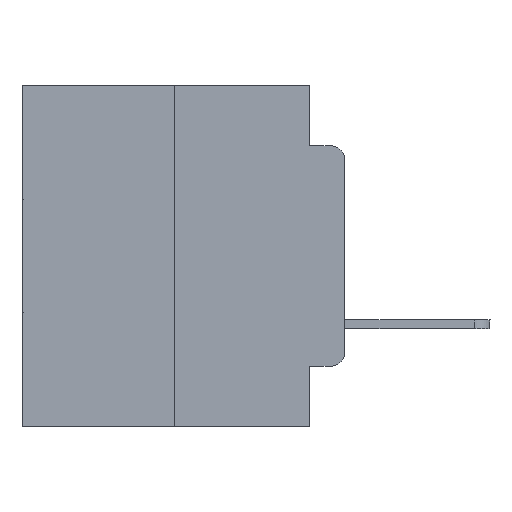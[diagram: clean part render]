
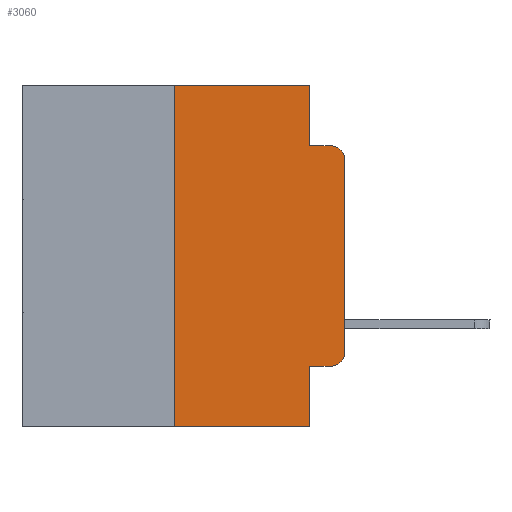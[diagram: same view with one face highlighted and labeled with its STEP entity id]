
A CAD part, left-side view. The second image highlights one B-rep face of the part: STEP entity #3060.
In plain terms, the highlighted planar face has unit normal (-1, 0, 0).
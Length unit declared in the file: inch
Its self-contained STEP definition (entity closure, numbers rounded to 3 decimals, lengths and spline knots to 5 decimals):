
#223 = DIRECTION ( 'NONE',  ( -1., 0., 0. ) ) ;
#539 = CARTESIAN_POINT ( 'NONE',  ( 0., 0.051, -0.0885 ) ) ;
#551 = VERTEX_POINT ( 'NONE', #13104 ) ;
#1118 = VERTEX_POINT ( 'NONE', #13674 ) ;
#1303 = DIRECTION ( 'NONE',  ( 0., -1., 0. ) ) ;
#1791 = CARTESIAN_POINT ( 'NONE',  ( 0., 0.25, 0. ) ) ;
#2303 = VERTEX_POINT ( 'NONE', #17810 ) ;
#2354 = VERTEX_POINT ( 'NONE', #6662 ) ;
#2661 = DIRECTION ( 'NONE',  ( 0., 0., -1. ) ) ;
#2842 = ORIENTED_EDGE ( 'NONE', *, *, #4212, .T. ) ;
#2928 = VECTOR ( 'NONE', #25773, 39.37008 ) ;
#2979 = EDGE_CURVE ( 'NONE', #2354, #1118, #25266, .T. ) ;
#3060 = ADVANCED_FACE ( 'NONE', ( #3319 ), #23708, .F. ) ;
#3319 = FACE_OUTER_BOUND ( 'NONE', #12115, .T. ) ;
#3343 = LINE ( 'NONE', #13105, #24347 ) ;
#3654 = VECTOR ( 'NONE', #1303, 39.37008 ) ;
#3935 = DIRECTION ( 'NONE',  ( 0., -1., 0. ) ) ;
#4157 = VECTOR ( 'NONE', #12078, 39.37008 ) ;
#4212 = EDGE_CURVE ( 'NONE', #8080, #551, #16313, .T. ) ;
#4447 = ORIENTED_EDGE ( 'NONE', *, *, #25679, .T. ) ;
#4883 = EDGE_CURVE ( 'NONE', #2303, #24372, #14687, .T. ) ;
#5353 = CARTESIAN_POINT ( 'NONE',  ( 0., 0.473, -0.5 ) ) ;
#5866 = CARTESIAN_POINT ( 'NONE',  ( 0., 0.051, -0.0885 ) ) ;
#6138 = ORIENTED_EDGE ( 'NONE', *, *, #2979, .F. ) ;
#6162 = DIRECTION ( 'NONE',  ( 0., 0., -1. ) ) ;
#6662 = CARTESIAN_POINT ( 'NONE',  ( 0., 0.051, -0.4115 ) ) ;
#6898 = DIRECTION ( 'NONE',  ( 0., 0., -1. ) ) ;
#8073 = CARTESIAN_POINT ( 'NONE',  ( 0., 0.473, 0. ) ) ;
#8080 = VERTEX_POINT ( 'NONE', #8433 ) ;
#8363 = AXIS2_PLACEMENT_3D ( 'NONE', #21636, #25627, #21457 ) ;
#8419 = CARTESIAN_POINT ( 'NONE',  ( 0., 0.02, -0.3915 ) ) ;
#8433 = CARTESIAN_POINT ( 'NONE',  ( 0., 0.02, -0.4115 ) ) ;
#8574 = CARTESIAN_POINT ( 'NONE',  ( 0., 0., -0.1085 ) ) ;
#8920 = ORIENTED_EDGE ( 'NONE', *, *, #13687, .T. ) ;
#9030 = ORIENTED_EDGE ( 'NONE', *, *, #18184, .F. ) ;
#9921 = VECTOR ( 'NONE', #12457, 39.37008 ) ;
#10866 = ORIENTED_EDGE ( 'NONE', *, *, #4883, .F. ) ;
#11330 = ORIENTED_EDGE ( 'NONE', *, *, #13579, .T. ) ;
#11761 = CARTESIAN_POINT ( 'NONE',  ( 0., 0.02, -0.0885 ) ) ;
#11883 = AXIS2_PLACEMENT_3D ( 'NONE', #8419, #223, #6162 ) ;
#11957 = LINE ( 'NONE', #17740, #3654 ) ;
#12078 = DIRECTION ( 'NONE',  ( 0., 0., 1. ) ) ;
#12115 = EDGE_LOOP ( 'NONE', ( #11330, #4447, #24808, #23043, #10866, #9030, #8920, #6138, #24757, #2842 ) ) ;
#12457 = DIRECTION ( 'NONE',  ( 0., -1., 0. ) ) ;
#12649 = EDGE_CURVE ( 'NONE', #24372, #23539, #3343, .T. ) ;
#13104 = CARTESIAN_POINT ( 'NONE',  ( 0., 0., -0.3915 ) ) ;
#13105 = CARTESIAN_POINT ( 'NONE',  ( 0., 0.051, 0. ) ) ;
#13303 = CIRCLE ( 'NONE', #8363, 0.02 ) ;
#13579 = EDGE_CURVE ( 'NONE', #551, #26294, #24578, .T. ) ;
#13674 = CARTESIAN_POINT ( 'NONE',  ( 0., 0.051, -0.5 ) ) ;
#13687 = EDGE_CURVE ( 'NONE', #20233, #1118, #21127, .T. ) ;
#14687 = LINE ( 'NONE', #8073, #9921 ) ;
#15639 = CARTESIAN_POINT ( 'NONE',  ( 0., 0.473, 0. ) ) ;
#15775 = CARTESIAN_POINT ( 'NONE',  ( 0., 0., 0. ) ) ;
#16161 = AXIS2_PLACEMENT_3D ( 'NONE', #15639, #25661, #19357 ) ;
#16313 = CIRCLE ( 'NONE', #11883, 0.02 ) ;
#16830 = LINE ( 'NONE', #5866, #21285 ) ;
#17740 = CARTESIAN_POINT ( 'NONE',  ( 0., 0.051, -0.4115 ) ) ;
#17810 = CARTESIAN_POINT ( 'NONE',  ( 0., 0.25, 0. ) ) ;
#18184 = EDGE_CURVE ( 'NONE', #20233, #2303, #22641, .T. ) ;
#18734 = VERTEX_POINT ( 'NONE', #11761 ) ;
#19357 = DIRECTION ( 'NONE',  ( 0., 0., -1. ) ) ;
#19499 = DIRECTION ( 'NONE',  ( 0., 0., 1. ) ) ;
#19988 = CARTESIAN_POINT ( 'NONE',  ( 0., 0.25, -0.5 ) ) ;
#20225 = VECTOR ( 'NONE', #2661, 39.37008 ) ;
#20233 = VERTEX_POINT ( 'NONE', #19988 ) ;
#21127 = LINE ( 'NONE', #5353, #2928 ) ;
#21285 = VECTOR ( 'NONE', #3935, 39.37008 ) ;
#21297 = EDGE_CURVE ( 'NONE', #23539, #18734, #16830, .T. ) ;
#21457 = DIRECTION ( 'NONE',  ( 0., 0., -1. ) ) ;
#21636 = CARTESIAN_POINT ( 'NONE',  ( 0., 0.02, -0.1085 ) ) ;
#22176 = EDGE_CURVE ( 'NONE', #2354, #8080, #11957, .T. ) ;
#22641 = LINE ( 'NONE', #1791, #4157 ) ;
#22983 = CARTESIAN_POINT ( 'NONE',  ( 0., 0.051, 0. ) ) ;
#23043 = ORIENTED_EDGE ( 'NONE', *, *, #12649, .F. ) ;
#23200 = CARTESIAN_POINT ( 'NONE',  ( 0., 0.051, 0. ) ) ;
#23539 = VERTEX_POINT ( 'NONE', #539 ) ;
#23708 = PLANE ( 'NONE',  #16161 ) ;
#24291 = VECTOR ( 'NONE', #19499, 39.37008 ) ;
#24347 = VECTOR ( 'NONE', #6898, 39.37008 ) ;
#24372 = VERTEX_POINT ( 'NONE', #23200 ) ;
#24578 = LINE ( 'NONE', #15775, #24291 ) ;
#24757 = ORIENTED_EDGE ( 'NONE', *, *, #22176, .T. ) ;
#24808 = ORIENTED_EDGE ( 'NONE', *, *, #21297, .F. ) ;
#25266 = LINE ( 'NONE', #22983, #20225 ) ;
#25627 = DIRECTION ( 'NONE',  ( -1., 0., 0. ) ) ;
#25661 = DIRECTION ( 'NONE',  ( 1., 0., 0. ) ) ;
#25679 = EDGE_CURVE ( 'NONE', #26294, #18734, #13303, .T. ) ;
#25773 = DIRECTION ( 'NONE',  ( 0., -1., 0. ) ) ;
#26294 = VERTEX_POINT ( 'NONE', #8574 ) ;
